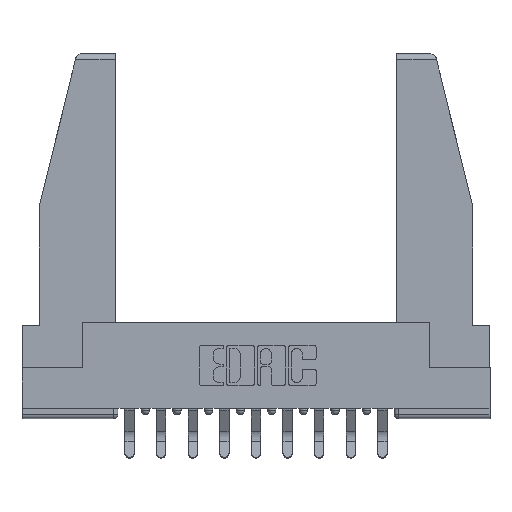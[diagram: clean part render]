
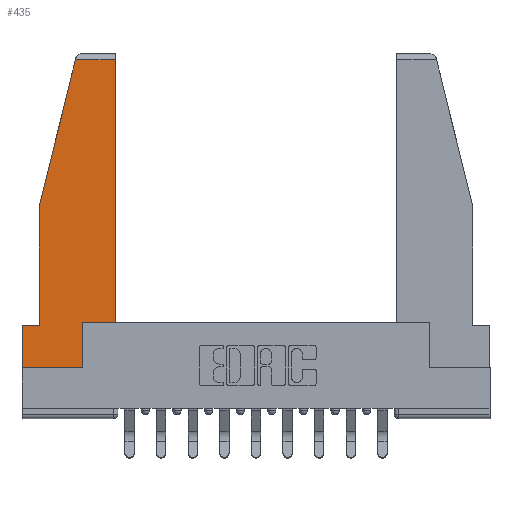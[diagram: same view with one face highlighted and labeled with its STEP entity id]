
A CAD part, top view. The second image highlights one B-rep face of the part: STEP entity #435.
In plain terms, the highlighted planar face has unit normal (0, 0, 1).
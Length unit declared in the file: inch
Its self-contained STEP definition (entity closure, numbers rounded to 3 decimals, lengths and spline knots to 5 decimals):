
#38 = EDGE_CURVE ( 'NONE', #14067, #8726, #7323, .T. ) ;
#172 = CARTESIAN_POINT ( 'NONE',  ( 0., 0., 0. ) ) ;
#435 = ADVANCED_FACE ( 'NONE', ( #4261 ), #6221, .T. ) ;
#458 = ORIENTED_EDGE ( 'NONE', *, *, #9813, .T. ) ;
#608 = CARTESIAN_POINT ( 'NONE',  ( 0.086, 0.8, 0. ) ) ;
#819 = EDGE_CURVE ( 'NONE', #3892, #14067, #2282, .T. ) ;
#868 = ORIENTED_EDGE ( 'NONE', *, *, #2585, .T. ) ;
#1480 = CARTESIAN_POINT ( 'NONE',  ( 0.297, 0., 0. ) ) ;
#1573 = VECTOR ( 'NONE', #6129, 39.37008 ) ;
#1692 = EDGE_CURVE ( 'NONE', #6655, #3892, #3522, .T. ) ;
#2282 = LINE ( 'NONE', #2361, #10984 ) ;
#2361 = CARTESIAN_POINT ( 'NONE',  ( 0.461, 0.223, 0. ) ) ;
#2379 = DIRECTION ( 'NONE',  ( 1., 0., 0. ) ) ;
#2585 = EDGE_CURVE ( 'NONE', #4258, #5664, #4557, .T. ) ;
#2746 = AXIS2_PLACEMENT_3D ( 'NONE', #8580, #14128, #7421 ) ;
#2869 = LINE ( 'NONE', #172, #10860 ) ;
#2894 = ORIENTED_EDGE ( 'NONE', *, *, #5253, .T. ) ;
#3324 = ORIENTED_EDGE ( 'NONE', *, *, #7099, .T. ) ;
#3522 = LINE ( 'NONE', #14056, #6880 ) ;
#3619 = DIRECTION ( 'NONE',  ( 0., 1., 0. ) ) ;
#3732 = EDGE_CURVE ( 'NONE', #10211, #6655, #14420, .T. ) ;
#3805 = ORIENTED_EDGE ( 'NONE', *, *, #819, .T. ) ;
#3892 = VERTEX_POINT ( 'NONE', #9230 ) ;
#4028 = DIRECTION ( 'NONE',  ( -1., 0., 0. ) ) ;
#4198 = CARTESIAN_POINT ( 'NONE',  ( 0.461, 1.52, 0. ) ) ;
#4258 = VERTEX_POINT ( 'NONE', #11851 ) ;
#4261 = FACE_OUTER_BOUND ( 'NONE', #7876, .T. ) ;
#4295 = ORIENTED_EDGE ( 'NONE', *, *, #38, .T. ) ;
#4307 = VECTOR ( 'NONE', #7270, 39.37008 ) ;
#4391 = EDGE_CURVE ( 'NONE', #13171, #4258, #13876, .T. ) ;
#4557 = LINE ( 'NONE', #10812, #12698 ) ;
#5164 = LINE ( 'NONE', #7774, #6951 ) ;
#5253 = EDGE_CURVE ( 'NONE', #12936, #10211, #2869, .T. ) ;
#5352 = DIRECTION ( 'NONE',  ( 1., 0., 0. ) ) ;
#5446 = CARTESIAN_POINT ( 'NONE',  ( 0.086, 0.8, 0. ) ) ;
#5664 = VERTEX_POINT ( 'NONE', #9279 ) ;
#5736 = VECTOR ( 'NONE', #13355, 39.37008 ) ;
#6129 = DIRECTION ( 'NONE',  ( 0., -1., 0. ) ) ;
#6201 = CARTESIAN_POINT ( 'NONE',  ( 0.2636, 1.52, 0. ) ) ;
#6221 = PLANE ( 'NONE',  #2746 ) ;
#6262 = CARTESIAN_POINT ( 'NONE',  ( 0., 0.21, 0. ) ) ;
#6655 = VERTEX_POINT ( 'NONE', #12615 ) ;
#6880 = VECTOR ( 'NONE', #5352, 39.37008 ) ;
#6938 = CARTESIAN_POINT ( 'NONE',  ( 0., 0., 0. ) ) ;
#6951 = VECTOR ( 'NONE', #9024, 39.37008 ) ;
#7099 = EDGE_CURVE ( 'NONE', #8726, #13171, #5164, .T. ) ;
#7220 = CARTESIAN_POINT ( 'NONE',  ( 0., 1.52, 0. ) ) ;
#7270 = DIRECTION ( 'NONE',  ( -1., 0., 0. ) ) ;
#7323 = LINE ( 'NONE', #7220, #4307 ) ;
#7421 = DIRECTION ( 'NONE',  ( 1., 0., 0. ) ) ;
#7699 = CARTESIAN_POINT ( 'NONE',  ( 0.297, 0., 0. ) ) ;
#7774 = CARTESIAN_POINT ( 'NONE',  ( 0.271, 1.55, 0. ) ) ;
#7876 = EDGE_LOOP ( 'NONE', ( #3805, #4295, #3324, #10252, #868, #458, #2894, #12913, #14061 ) ) ;
#7945 = LINE ( 'NONE', #6262, #1573 ) ;
#8580 = CARTESIAN_POINT ( 'NONE',  ( 0., 0., 0. ) ) ;
#8726 = VERTEX_POINT ( 'NONE', #6201 ) ;
#9024 = DIRECTION ( 'NONE',  ( -0.239, -0.971, 0. ) ) ;
#9230 = CARTESIAN_POINT ( 'NONE',  ( 0.461, 0.223, 0. ) ) ;
#9279 = CARTESIAN_POINT ( 'NONE',  ( 0., 0.21, 0. ) ) ;
#9813 = EDGE_CURVE ( 'NONE', #5664, #12936, #7945, .T. ) ;
#10211 = VERTEX_POINT ( 'NONE', #1480 ) ;
#10252 = ORIENTED_EDGE ( 'NONE', *, *, #4391, .T. ) ;
#10812 = CARTESIAN_POINT ( 'NONE',  ( 0., 0.21, 0. ) ) ;
#10860 = VECTOR ( 'NONE', #2379, 39.37008 ) ;
#10984 = VECTOR ( 'NONE', #3619, 39.37008 ) ;
#11851 = CARTESIAN_POINT ( 'NONE',  ( 0.086, 0.21, 0. ) ) ;
#11963 = VECTOR ( 'NONE', #14261, 39.37008 ) ;
#12615 = CARTESIAN_POINT ( 'NONE',  ( 0.297, 0.223, 0. ) ) ;
#12698 = VECTOR ( 'NONE', #4028, 39.37008 ) ;
#12913 = ORIENTED_EDGE ( 'NONE', *, *, #3732, .T. ) ;
#12936 = VERTEX_POINT ( 'NONE', #6938 ) ;
#13171 = VERTEX_POINT ( 'NONE', #608 ) ;
#13355 = DIRECTION ( 'NONE',  ( 0., -1., 0. ) ) ;
#13876 = LINE ( 'NONE', #5446, #5736 ) ;
#14056 = CARTESIAN_POINT ( 'NONE',  ( 0.297, 0.223, 0. ) ) ;
#14061 = ORIENTED_EDGE ( 'NONE', *, *, #1692, .T. ) ;
#14067 = VERTEX_POINT ( 'NONE', #4198 ) ;
#14128 = DIRECTION ( 'NONE',  ( 0., 0., 1. ) ) ;
#14261 = DIRECTION ( 'NONE',  ( 0., 1., 0. ) ) ;
#14420 = LINE ( 'NONE', #7699, #11963 ) ;
